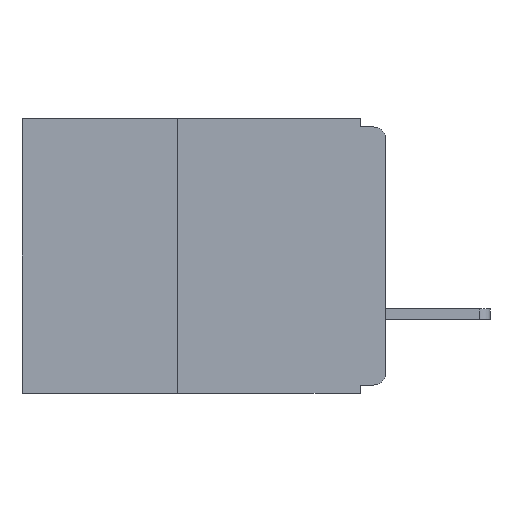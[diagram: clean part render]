
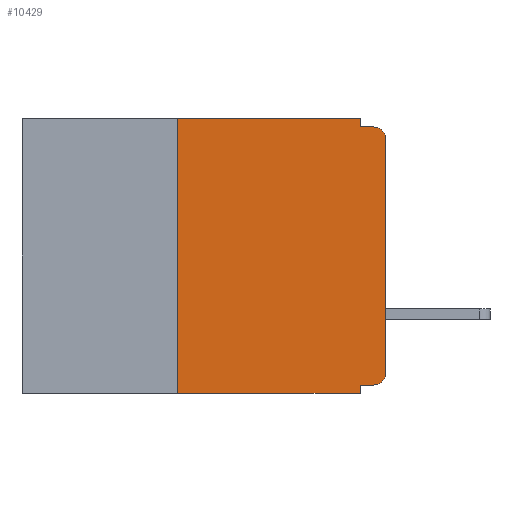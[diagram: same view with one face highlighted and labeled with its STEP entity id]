
A CAD part, left-side view. The second image highlights one B-rep face of the part: STEP entity #10429.
In plain terms, the highlighted planar face has unit normal (-1, 0, 0).
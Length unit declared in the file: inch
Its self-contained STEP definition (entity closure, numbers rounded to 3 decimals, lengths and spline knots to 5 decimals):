
#22 = LINE ( 'NONE', #13358, #6377 ) ;
#87 = CARTESIAN_POINT ( 'NONE',  ( 0., 0., -0.025 ) ) ;
#556 = DIRECTION ( 'NONE',  ( 0., 0., -1. ) ) ;
#730 = DIRECTION ( 'NONE',  ( 0., 0., -1. ) ) ;
#835 = VECTOR ( 'NONE', #1801, 39.37008 ) ;
#836 = DIRECTION ( 'NONE',  ( 0., 0., 1. ) ) ;
#879 = CARTESIAN_POINT ( 'NONE',  ( 0., 0.25, -0.33 ) ) ;
#920 = LINE ( 'NONE', #7320, #3557 ) ;
#928 = CARTESIAN_POINT ( 'NONE',  ( 0., 0.015, -0.305 ) ) ;
#1166 = AXIS2_PLACEMENT_3D ( 'NONE', #14616, #8038, #556 ) ;
#1280 = CARTESIAN_POINT ( 'NONE',  ( 0., 0.031, -0.01 ) ) ;
#1329 = VERTEX_POINT ( 'NONE', #5586 ) ;
#1735 = LINE ( 'NONE', #8393, #4334 ) ;
#1801 = DIRECTION ( 'NONE',  ( 0., 0., 1. ) ) ;
#1829 = CIRCLE ( 'NONE', #1166, 0.015 ) ;
#1973 = EDGE_CURVE ( 'NONE', #6852, #7486, #6381, .T. ) ;
#1995 = EDGE_LOOP ( 'NONE', ( #3091, #2083, #4763, #10449, #5725, #2894, #2657, #11017, #4675, #11033 ) ) ;
#2083 = ORIENTED_EDGE ( 'NONE', *, *, #10105, .T. ) ;
#2126 = LINE ( 'NONE', #8293, #5128 ) ;
#2209 = FACE_OUTER_BOUND ( 'NONE', #1995, .T. ) ;
#2221 = DIRECTION ( 'NONE',  ( 0., 0., -1. ) ) ;
#2554 = VECTOR ( 'NONE', #730, 39.37008 ) ;
#2657 = ORIENTED_EDGE ( 'NONE', *, *, #12451, .T. ) ;
#2663 = CARTESIAN_POINT ( 'NONE',  ( 0., 0.015, -0.01 ) ) ;
#2894 = ORIENTED_EDGE ( 'NONE', *, *, #12396, .F. ) ;
#3091 = ORIENTED_EDGE ( 'NONE', *, *, #9555, .T. ) ;
#3557 = VECTOR ( 'NONE', #8494, 39.37008 ) ;
#3862 = LINE ( 'NONE', #9170, #835 ) ;
#3912 = DIRECTION ( 'NONE',  ( 0., 0., -1. ) ) ;
#3956 = CARTESIAN_POINT ( 'NONE',  ( 0., 0.015, -0.32 ) ) ;
#4334 = VECTOR ( 'NONE', #4741, 39.37008 ) ;
#4675 = ORIENTED_EDGE ( 'NONE', *, *, #9999, .F. ) ;
#4738 = DIRECTION ( 'NONE',  ( 0., -1., 0. ) ) ;
#4741 = DIRECTION ( 'NONE',  ( 0., -1., 0. ) ) ;
#4763 = ORIENTED_EDGE ( 'NONE', *, *, #9757, .F. ) ;
#5112 = CARTESIAN_POINT ( 'NONE',  ( 0., 0., -0.305 ) ) ;
#5128 = VECTOR ( 'NONE', #836, 39.37008 ) ;
#5586 = CARTESIAN_POINT ( 'NONE',  ( 0., 0.031, -0.33 ) ) ;
#5725 = ORIENTED_EDGE ( 'NONE', *, *, #1973, .F. ) ;
#6377 = VECTOR ( 'NONE', #7784, 39.37008 ) ;
#6381 = LINE ( 'NONE', #7757, #12113 ) ;
#6406 = VERTEX_POINT ( 'NONE', #7382 ) ;
#6852 = VERTEX_POINT ( 'NONE', #10492 ) ;
#6908 = VERTEX_POINT ( 'NONE', #879 ) ;
#7181 = VERTEX_POINT ( 'NONE', #87 ) ;
#7320 = CARTESIAN_POINT ( 'NONE',  ( 0., 0.031, -0.33 ) ) ;
#7382 = CARTESIAN_POINT ( 'NONE',  ( 0., 0.031, -0.32 ) ) ;
#7486 = VERTEX_POINT ( 'NONE', #9433 ) ;
#7662 = DIRECTION ( 'NONE',  ( 0., -1., 0. ) ) ;
#7687 = VERTEX_POINT ( 'NONE', #5112 ) ;
#7757 = CARTESIAN_POINT ( 'NONE',  ( 0., 0.437, 0. ) ) ;
#7784 = DIRECTION ( 'NONE',  ( 0., 1., 0. ) ) ;
#8038 = DIRECTION ( 'NONE',  ( -1., 0., 0. ) ) ;
#8293 = CARTESIAN_POINT ( 'NONE',  ( 0., 0.25, -0.33 ) ) ;
#8393 = CARTESIAN_POINT ( 'NONE',  ( 0., 0.437, -0.33 ) ) ;
#8494 = DIRECTION ( 'NONE',  ( 0., 0., -1. ) ) ;
#8554 = AXIS2_PLACEMENT_3D ( 'NONE', #8744, #11010, #3912 ) ;
#8579 = CIRCLE ( 'NONE', #10920, 0.015 ) ;
#8744 = CARTESIAN_POINT ( 'NONE',  ( 0., 0.437, 0. ) ) ;
#9170 = CARTESIAN_POINT ( 'NONE',  ( 0., 0., 0. ) ) ;
#9296 = CARTESIAN_POINT ( 'NONE',  ( 0., 0.031, 0. ) ) ;
#9433 = CARTESIAN_POINT ( 'NONE',  ( 0., 0.031, 0. ) ) ;
#9535 = DIRECTION ( 'NONE',  ( -1., 0., 0. ) ) ;
#9555 = EDGE_CURVE ( 'NONE', #7687, #7181, #3862, .T. ) ;
#9757 = EDGE_CURVE ( 'NONE', #14684, #12682, #10385, .T. ) ;
#9999 = EDGE_CURVE ( 'NONE', #12034, #6406, #22, .T. ) ;
#10105 = EDGE_CURVE ( 'NONE', #7181, #12682, #1829, .T. ) ;
#10254 = EDGE_CURVE ( 'NONE', #12034, #7687, #8579, .T. ) ;
#10385 = LINE ( 'NONE', #12825, #11094 ) ;
#10429 = ADVANCED_FACE ( 'NONE', ( #2209 ), #14211, .F. ) ;
#10449 = ORIENTED_EDGE ( 'NONE', *, *, #12347, .F. ) ;
#10492 = CARTESIAN_POINT ( 'NONE',  ( 0., 0.25, 0. ) ) ;
#10920 = AXIS2_PLACEMENT_3D ( 'NONE', #928, #9535, #2221 ) ;
#11010 = DIRECTION ( 'NONE',  ( 1., 0., 0. ) ) ;
#11017 = ORIENTED_EDGE ( 'NONE', *, *, #12495, .F. ) ;
#11033 = ORIENTED_EDGE ( 'NONE', *, *, #10254, .T. ) ;
#11094 = VECTOR ( 'NONE', #4738, 39.37008 ) ;
#12025 = LINE ( 'NONE', #9296, #2554 ) ;
#12034 = VERTEX_POINT ( 'NONE', #3956 ) ;
#12113 = VECTOR ( 'NONE', #7662, 39.37008 ) ;
#12347 = EDGE_CURVE ( 'NONE', #7486, #14684, #12025, .T. ) ;
#12396 = EDGE_CURVE ( 'NONE', #6908, #6852, #2126, .T. ) ;
#12451 = EDGE_CURVE ( 'NONE', #6908, #1329, #1735, .T. ) ;
#12495 = EDGE_CURVE ( 'NONE', #6406, #1329, #920, .T. ) ;
#12682 = VERTEX_POINT ( 'NONE', #2663 ) ;
#12825 = CARTESIAN_POINT ( 'NONE',  ( 0., 0., -0.01 ) ) ;
#13358 = CARTESIAN_POINT ( 'NONE',  ( 0., 0., -0.32 ) ) ;
#14211 = PLANE ( 'NONE',  #8554 ) ;
#14616 = CARTESIAN_POINT ( 'NONE',  ( 0., 0.015, -0.025 ) ) ;
#14684 = VERTEX_POINT ( 'NONE', #1280 ) ;
